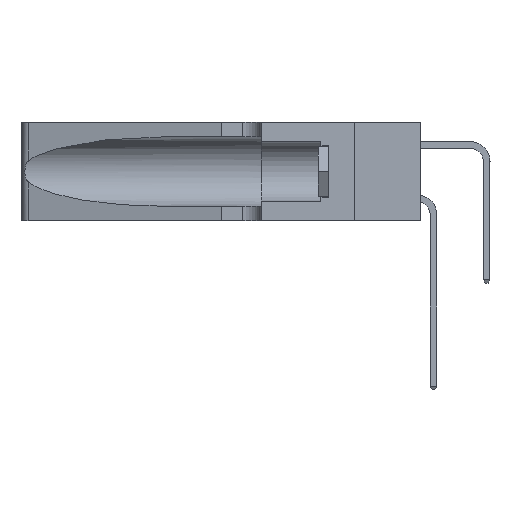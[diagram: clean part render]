
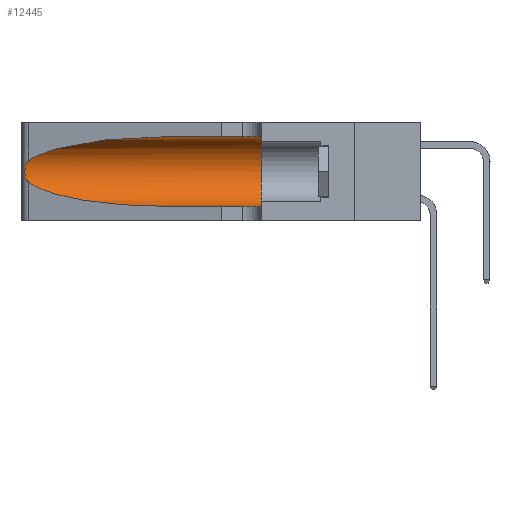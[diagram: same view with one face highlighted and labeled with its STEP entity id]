
A CAD part, left-side view. The second image highlights one B-rep face of the part: STEP entity #12445.
In plain terms, the highlighted cylindrical face has radius 3.308 mm (diameter 6.617 mm), a partial arc.
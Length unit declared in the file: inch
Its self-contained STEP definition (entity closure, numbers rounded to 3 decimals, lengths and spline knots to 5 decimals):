
#1476 = LINE ( 'NONE', #18831, #21774 ) ;
#1693 = DIRECTION ( 'NONE',  ( 0., 1., 0. ) ) ;
#2642 = CARTESIAN_POINT ( 'NONE',  ( 0.25639, 1.23186, 0.15144 ) ) ;
#2806 = EDGE_CURVE ( 'NONE', #4990, #26192, #1476, .T. ) ;
#4801 = ORIENTED_EDGE ( 'NONE', *, *, #32416, .T. ) ;
#4862 = EDGE_LOOP ( 'NONE', ( #4801, #8329, #14855, #29656, #16502, #23348 ) ) ;
#4990 = VERTEX_POINT ( 'NONE', #30074 ) ;
#5305 = CARTESIAN_POINT ( 'NONE',  ( 0.25487, 1.22718, 0.14631 ) ) ;
#6459 = CARTESIAN_POINT ( 'NONE',  ( 0.2373, 1.15595, 0.28018 ) ) ;
#6461 = DIRECTION ( 'NONE',  ( 0., 0., -1. ) ) ;
#6601 = CARTESIAN_POINT ( 'NONE',  ( 0.1305, 1.61858, 0.31525 ) ) ;
#7761 = EDGE_CURVE ( 'NONE', #30778, #4990, #9431, .T. ) ;
#7772 = CARTESIAN_POINT ( 'NONE',  ( 0.25487, 1.22718, 0.22369 ) ) ;
#7836 = CARTESIAN_POINT ( 'NONE',  ( 0.25639, 1.23184, 0.21858 ) ) ;
#8329 = ORIENTED_EDGE ( 'NONE', *, *, #14832, .T. ) ;
#9431 =( BOUNDED_CURVE ( )  B_SPLINE_CURVE ( 3, ( #21524, #26678, #10987, #29412 ),
 .UNSPECIFIED., .F., .T. ) 
 B_SPLINE_CURVE_WITH_KNOTS ( ( 4, 4 ),
 ( 3.44316, 4.71239 ),
 .UNSPECIFIED. ) 
 CURVE ( )  GEOMETRIC_REPRESENTATION_ITEM ( )  RATIONAL_B_SPLINE_CURVE ( ( 1., 0.87, 0.87, 1. ) ) 
 REPRESENTATION_ITEM ( '' )  );
#9777 = CARTESIAN_POINT ( 'NONE',  ( 0.1305, 0.35, 0.05475 ) ) ;
#10226 = AXIS2_PLACEMENT_3D ( 'NONE', #17046, #22363, #6461 ) ;
#10519 = CARTESIAN_POINT ( 'NONE',  ( 0.25854, 1.2359, 0.20912 ) ) ;
#10624 = VERTEX_POINT ( 'NONE', #28078 ) ;
#10987 = CARTESIAN_POINT ( 'NONE',  ( 0.18966, 0.96281, 0.05475 ) ) ;
#11838 = DIRECTION ( 'NONE',  ( 0., -1., 0. ) ) ;
#12445 = ADVANCED_FACE ( 'NONE', ( #14751 ), #34069, .F. ) ;
#12477 = VERTEX_POINT ( 'NONE', #25107 ) ;
#13068 = B_SPLINE_CURVE_WITH_KNOTS ( 'NONE', 3,
 ( #21043, #23721, #7836, #26322, #10519, #28954, #13184, #31611, #15864, #22794, #18510, #2642, #21161, #5305 ),
 .UNSPECIFIED., .F., .F.,
 ( 4, 2, 2, 2, 2, 2, 4 ),
 ( 0., 0.00027, 0.00053, 0.00107, 0.0016, 0.00187, 0.00214 ),
 .UNSPECIFIED. ) ;
#13184 = CARTESIAN_POINT ( 'NONE',  ( 0.26075, 1.23896, 0.19203 ) ) ;
#13222 = CIRCLE ( 'NONE', #24880, 0.13025 ) ;
#14379 = CARTESIAN_POINT ( 'NONE',  ( 0.18966, 0.96281, 0.31525 ) ) ;
#14751 = FACE_OUTER_BOUND ( 'NONE', #4862, .T. ) ;
#14832 = EDGE_CURVE ( 'NONE', #30081, #30778, #13068, .T. ) ;
#14855 = ORIENTED_EDGE ( 'NONE', *, *, #7761, .T. ) ;
#15864 = CARTESIAN_POINT ( 'NONE',  ( 0.26017, 1.23833, 0.17102 ) ) ;
#16502 = ORIENTED_EDGE ( 'NONE', *, *, #24116, .F. ) ;
#16610 = EDGE_CURVE ( 'NONE', #10624, #12477, #29312, .T. ) ;
#17045 = CARTESIAN_POINT ( 'NONE',  ( 0.1305, 0.72297, 0.31525 ) ) ;
#17046 = CARTESIAN_POINT ( 'NONE',  ( 0.1305, 1.61858, 0.185 ) ) ;
#17571 = CARTESIAN_POINT ( 'NONE',  ( 0.1305, 0.35, 0.185 ) ) ;
#18510 = CARTESIAN_POINT ( 'NONE',  ( 0.25789, 1.23486, 0.15765 ) ) ;
#18831 = CARTESIAN_POINT ( 'NONE',  ( 0.1305, 1.61858, 0.05475 ) ) ;
#20214 = DIRECTION ( 'NONE',  ( 0., 0., 1. ) ) ;
#20261 =( BOUNDED_CURVE ( )  B_SPLINE_CURVE ( 3, ( #17045, #14379, #6459, #24990 ),
 .UNSPECIFIED., .F., .F. ) 
 B_SPLINE_CURVE_WITH_KNOTS ( ( 4, 4 ),
 ( 1.5708, 2.84003 ),
 .UNSPECIFIED. ) 
 CURVE ( )  GEOMETRIC_REPRESENTATION_ITEM ( )  RATIONAL_B_SPLINE_CURVE ( ( 1., 0.87, 0.87, 1. ) ) 
 REPRESENTATION_ITEM ( '' )  );
#21043 = CARTESIAN_POINT ( 'NONE',  ( 0.25487, 1.22718, 0.22369 ) ) ;
#21048 = CARTESIAN_POINT ( 'NONE',  ( 0.25487, 1.22718, 0.14631 ) ) ;
#21161 = CARTESIAN_POINT ( 'NONE',  ( 0.25555, 1.22993, 0.14849 ) ) ;
#21524 = CARTESIAN_POINT ( 'NONE',  ( 0.25487, 1.22718, 0.14631 ) ) ;
#21774 = VECTOR ( 'NONE', #24173, 39.37008 ) ;
#22363 = DIRECTION ( 'NONE',  ( 0., -1., 0. ) ) ;
#22794 = CARTESIAN_POINT ( 'NONE',  ( 0.25856, 1.23593, 0.16098 ) ) ;
#23197 = VECTOR ( 'NONE', #11838, 39.37008 ) ;
#23348 = ORIENTED_EDGE ( 'NONE', *, *, #16610, .F. ) ;
#23721 = CARTESIAN_POINT ( 'NONE',  ( 0.25555, 1.22994, 0.2215 ) ) ;
#24116 = EDGE_CURVE ( 'NONE', #12477, #26192, #13222, .T. ) ;
#24173 = DIRECTION ( 'NONE',  ( 0., -1., 0. ) ) ;
#24880 = AXIS2_PLACEMENT_3D ( 'NONE', #17571, #1693, #20214 ) ;
#24990 = CARTESIAN_POINT ( 'NONE',  ( 0.25487, 1.22718, 0.22369 ) ) ;
#25107 = CARTESIAN_POINT ( 'NONE',  ( 0.1305, 0.35, 0.31525 ) ) ;
#26192 = VERTEX_POINT ( 'NONE', #9777 ) ;
#26322 = CARTESIAN_POINT ( 'NONE',  ( 0.25787, 1.23484, 0.2124 ) ) ;
#26678 = CARTESIAN_POINT ( 'NONE',  ( 0.2373, 1.15595, 0.08982 ) ) ;
#28078 = CARTESIAN_POINT ( 'NONE',  ( 0.1305, 0.72297, 0.31525 ) ) ;
#28954 = CARTESIAN_POINT ( 'NONE',  ( 0.26018, 1.23835, 0.19895 ) ) ;
#29312 = LINE ( 'NONE', #6601, #23197 ) ;
#29412 = CARTESIAN_POINT ( 'NONE',  ( 0.1305, 0.72297, 0.05475 ) ) ;
#29656 = ORIENTED_EDGE ( 'NONE', *, *, #2806, .T. ) ;
#30074 = CARTESIAN_POINT ( 'NONE',  ( 0.1305, 0.72297, 0.05475 ) ) ;
#30081 = VERTEX_POINT ( 'NONE', #7772 ) ;
#30778 = VERTEX_POINT ( 'NONE', #21048 ) ;
#31611 = CARTESIAN_POINT ( 'NONE',  ( 0.26075, 1.23896, 0.178 ) ) ;
#32416 = EDGE_CURVE ( 'NONE', #10624, #30081, #20261, .T. ) ;
#34069 = CYLINDRICAL_SURFACE ( 'NONE', #10226, 0.13025 ) ;
